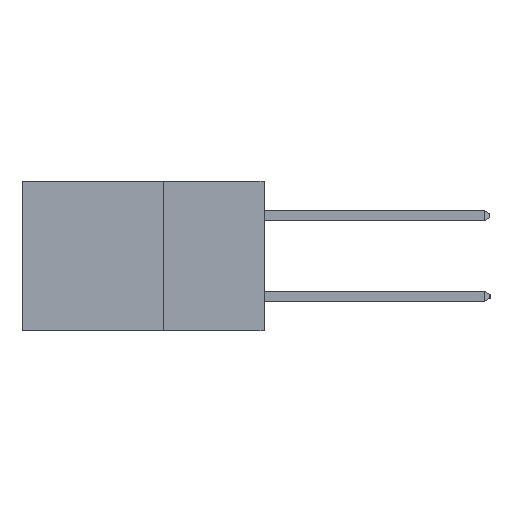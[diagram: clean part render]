
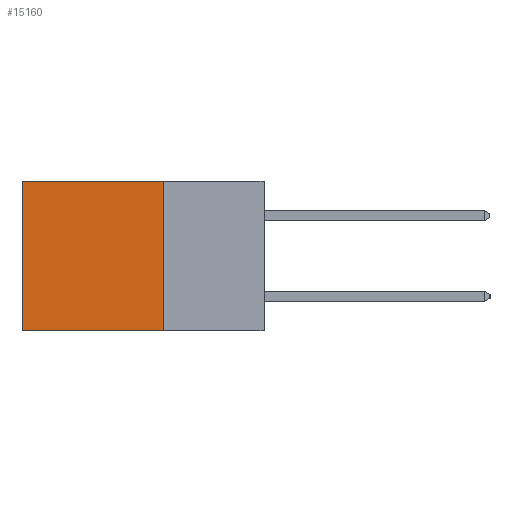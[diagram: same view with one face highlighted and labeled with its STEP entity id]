
A CAD part, left-side view. The second image highlights one B-rep face of the part: STEP entity #15160.
In plain terms, the highlighted planar face has unit normal (-1, 0, 0).
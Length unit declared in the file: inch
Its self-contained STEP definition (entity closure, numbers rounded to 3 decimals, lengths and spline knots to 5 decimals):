
#83 = DIRECTION ( 'NONE',  ( 0., 0., -1. ) ) ;
#1142 = LINE ( 'NONE', #2488, #6967 ) ;
#1377 = CARTESIAN_POINT ( 'NONE',  ( 0.2615, 0.6, -0.37 ) ) ;
#2403 = CARTESIAN_POINT ( 'NONE',  ( 0.2615, 0.25, -0.37 ) ) ;
#2413 = VERTEX_POINT ( 'NONE', #1377 ) ;
#2488 = CARTESIAN_POINT ( 'NONE',  ( 0.2615, 0.25, -0.37 ) ) ;
#2917 = EDGE_CURVE ( 'NONE', #13983, #5133, #1142, .T. ) ;
#3463 = EDGE_LOOP ( 'NONE', ( #7866, #12285, #11819, #10650 ) ) ;
#3586 = DIRECTION ( 'NONE',  ( 0., 1., 0. ) ) ;
#3989 = AXIS2_PLACEMENT_3D ( 'NONE', #12989, #7068, #83 ) ;
#4720 = PLANE ( 'NONE',  #3989 ) ;
#5133 = VERTEX_POINT ( 'NONE', #14609 ) ;
#5768 = VECTOR ( 'NONE', #14520, 39.37008 ) ;
#5933 = EDGE_CURVE ( 'NONE', #13201, #2413, #14152, .T. ) ;
#6554 = CARTESIAN_POINT ( 'NONE',  ( 0.2615, 0.6, -0.37 ) ) ;
#6967 = VECTOR ( 'NONE', #10642, 39.37008 ) ;
#7068 = DIRECTION ( 'NONE',  ( 1., 0., 0. ) ) ;
#7866 = ORIENTED_EDGE ( 'NONE', *, *, #5933, .T. ) ;
#8294 = EDGE_CURVE ( 'NONE', #13983, #13201, #12811, .T. ) ;
#8815 = CARTESIAN_POINT ( 'NONE',  ( 0.2615, 0.6, 0. ) ) ;
#10642 = DIRECTION ( 'NONE',  ( 0., 0., -1. ) ) ;
#10650 = ORIENTED_EDGE ( 'NONE', *, *, #8294, .T. ) ;
#10958 = VECTOR ( 'NONE', #14842, 39.37008 ) ;
#11093 = EDGE_CURVE ( 'NONE', #5133, #2413, #12268, .T. ) ;
#11819 = ORIENTED_EDGE ( 'NONE', *, *, #2917, .F. ) ;
#11887 = VECTOR ( 'NONE', #3586, 39.37008 ) ;
#12268 = LINE ( 'NONE', #2403, #11887 ) ;
#12285 = ORIENTED_EDGE ( 'NONE', *, *, #11093, .F. ) ;
#12337 = FACE_OUTER_BOUND ( 'NONE', #3463, .T. ) ;
#12632 = CARTESIAN_POINT ( 'NONE',  ( 0.2615, 0.25, 0. ) ) ;
#12811 = LINE ( 'NONE', #13360, #5768 ) ;
#12989 = CARTESIAN_POINT ( 'NONE',  ( 0.2615, 0.25, -0.37 ) ) ;
#13201 = VERTEX_POINT ( 'NONE', #8815 ) ;
#13360 = CARTESIAN_POINT ( 'NONE',  ( 0.2615, 0.25, 0. ) ) ;
#13983 = VERTEX_POINT ( 'NONE', #12632 ) ;
#14152 = LINE ( 'NONE', #6554, #10958 ) ;
#14520 = DIRECTION ( 'NONE',  ( 0., 1., 0. ) ) ;
#14609 = CARTESIAN_POINT ( 'NONE',  ( 0.2615, 0.25, -0.37 ) ) ;
#14842 = DIRECTION ( 'NONE',  ( 0., 0., -1. ) ) ;
#15160 = ADVANCED_FACE ( 'NONE', ( #12337 ), #4720, .F. ) ;
